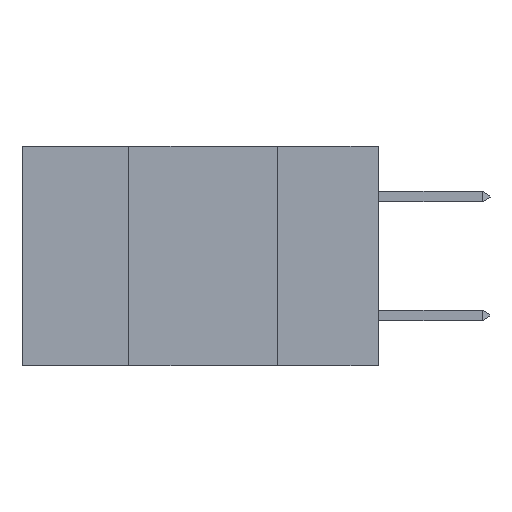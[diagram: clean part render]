
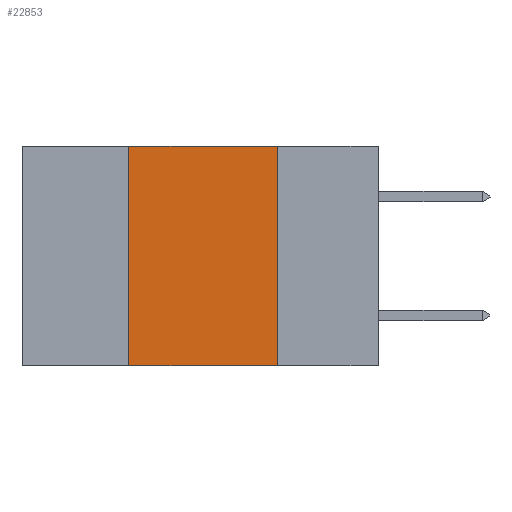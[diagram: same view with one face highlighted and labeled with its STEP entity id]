
A CAD part, left-side view. The second image highlights one B-rep face of the part: STEP entity #22853.
In plain terms, the highlighted planar face has unit normal (-1, 0, 0).
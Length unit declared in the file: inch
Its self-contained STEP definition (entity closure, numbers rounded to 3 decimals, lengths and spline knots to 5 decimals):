
#2286 = CARTESIAN_POINT ( 'NONE',  ( 0., 0.6, -0.37 ) ) ;
#3272 = CARTESIAN_POINT ( 'NONE',  ( 0., 0.42, -0.37 ) ) ;
#3475 = DIRECTION ( 'NONE',  ( 1., 0., 0. ) ) ;
#4059 = DIRECTION ( 'NONE',  ( 0., 0., 1. ) ) ;
#4087 = CARTESIAN_POINT ( 'NONE',  ( 0., 0.17, 0. ) ) ;
#4095 = DIRECTION ( 'NONE',  ( 0., -1., 0. ) ) ;
#5599 = CARTESIAN_POINT ( 'NONE',  ( 0., 0.42, 0. ) ) ;
#5766 = EDGE_CURVE ( 'NONE', #8388, #7075, #11245, .T. ) ;
#5998 = FACE_OUTER_BOUND ( 'NONE', #17481, .T. ) ;
#6000 = EDGE_CURVE ( 'NONE', #22094, #7162, #20853, .T. ) ;
#6123 = VECTOR ( 'NONE', #4059, 39.37008 ) ;
#6463 = VECTOR ( 'NONE', #16090, 39.37008 ) ;
#7075 = VERTEX_POINT ( 'NONE', #22773 ) ;
#7162 = VERTEX_POINT ( 'NONE', #15959 ) ;
#8388 = VERTEX_POINT ( 'NONE', #5599 ) ;
#9664 = ORIENTED_EDGE ( 'NONE', *, *, #5766, .F. ) ;
#10661 = EDGE_CURVE ( 'NONE', #22094, #8388, #15065, .T. ) ;
#11245 = LINE ( 'NONE', #19510, #6463 ) ;
#11520 = VECTOR ( 'NONE', #4095, 39.37008 ) ;
#11714 = VECTOR ( 'NONE', #18406, 39.37008 ) ;
#13030 = CARTESIAN_POINT ( 'NONE',  ( 0., 0.42, 0. ) ) ;
#13982 = AXIS2_PLACEMENT_3D ( 'NONE', #21191, #3475, #15997 ) ;
#14246 = PLANE ( 'NONE',  #13982 ) ;
#14426 = ORIENTED_EDGE ( 'NONE', *, *, #10661, .F. ) ;
#14975 = ORIENTED_EDGE ( 'NONE', *, *, #6000, .T. ) ;
#15065 = LINE ( 'NONE', #13030, #6123 ) ;
#15251 = EDGE_CURVE ( 'NONE', #7075, #7162, #16402, .T. ) ;
#15959 = CARTESIAN_POINT ( 'NONE',  ( 0., 0.17, -0.37 ) ) ;
#15997 = DIRECTION ( 'NONE',  ( 0., 0., -1. ) ) ;
#16090 = DIRECTION ( 'NONE',  ( 0., -1., 0. ) ) ;
#16402 = LINE ( 'NONE', #4087, #11714 ) ;
#17481 = EDGE_LOOP ( 'NONE', ( #17977, #9664, #14426, #14975 ) ) ;
#17977 = ORIENTED_EDGE ( 'NONE', *, *, #15251, .F. ) ;
#18406 = DIRECTION ( 'NONE',  ( 0., 0., -1. ) ) ;
#19510 = CARTESIAN_POINT ( 'NONE',  ( 0., 0.6, 0. ) ) ;
#20853 = LINE ( 'NONE', #2286, #11520 ) ;
#21191 = CARTESIAN_POINT ( 'NONE',  ( 0., 0.6, 0. ) ) ;
#22094 = VERTEX_POINT ( 'NONE', #3272 ) ;
#22773 = CARTESIAN_POINT ( 'NONE',  ( 0., 0.17, 0. ) ) ;
#22853 = ADVANCED_FACE ( 'NONE', ( #5998 ), #14246, .F. ) ;
